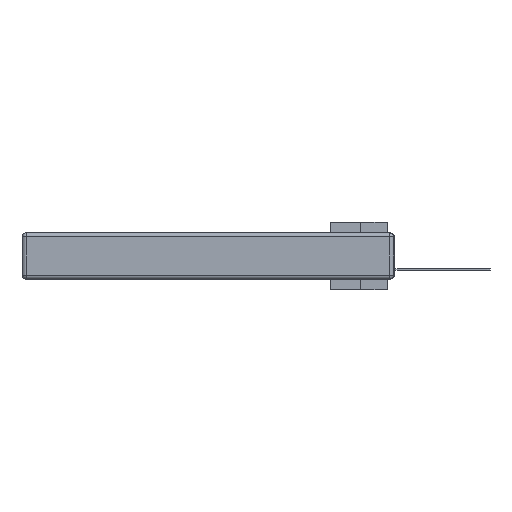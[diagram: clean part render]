
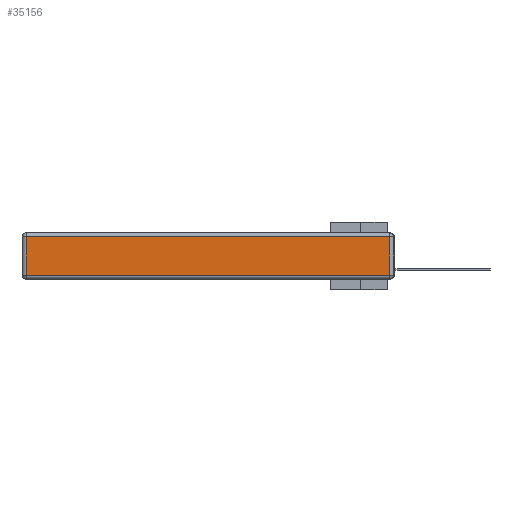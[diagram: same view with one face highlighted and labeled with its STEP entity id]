
A CAD part, left-side view. The second image highlights one B-rep face of the part: STEP entity #35156.
In plain terms, the highlighted planar face has unit normal (-1, 0, 0).
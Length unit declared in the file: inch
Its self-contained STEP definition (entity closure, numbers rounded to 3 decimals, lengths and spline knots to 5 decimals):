
#4 = EDGE_LOOP ( 'NONE', ( #25495, #147, #32077, #815 ) ) ;
#147 = ORIENTED_EDGE ( 'NONE', *, *, #21428, .T. ) ;
#815 = ORIENTED_EDGE ( 'NONE', *, *, #32978, .T. ) ;
#996 = LINE ( 'NONE', #24445, #1953 ) ;
#1953 = VECTOR ( 'NONE', #3888, 39.37008 ) ;
#2244 = AXIS2_PLACEMENT_3D ( 'NONE', #6804, #35891, #18681 ) ;
#3125 = CARTESIAN_POINT ( 'NONE',  ( 0., 2.72, -0.313 ) ) ;
#3888 = DIRECTION ( 'NONE',  ( 0., 1., 0. ) ) ;
#5013 = VECTOR ( 'NONE', #20433, 39.37008 ) ;
#5311 = CARTESIAN_POINT ( 'NONE',  ( 0., 0.03, -0.343 ) ) ;
#6804 = CARTESIAN_POINT ( 'NONE',  ( 0., 0., -0.343 ) ) ;
#7514 = LINE ( 'NONE', #17478, #15366 ) ;
#7903 = CARTESIAN_POINT ( 'NONE',  ( 0., 0.03, -0.313 ) ) ;
#8683 = VERTEX_POINT ( 'NONE', #11463 ) ;
#10481 = FACE_OUTER_BOUND ( 'NONE', #4, .T. ) ;
#11463 = CARTESIAN_POINT ( 'NONE',  ( 0., 0.03, -0.03 ) ) ;
#13597 = EDGE_CURVE ( 'NONE', #29920, #30816, #7514, .T. ) ;
#15366 = VECTOR ( 'NONE', #32072, 39.37008 ) ;
#15825 = VERTEX_POINT ( 'NONE', #30390 ) ;
#17478 = CARTESIAN_POINT ( 'NONE',  ( 0., 0., -0.313 ) ) ;
#18681 = DIRECTION ( 'NONE',  ( 0., 0., 1. ) ) ;
#20433 = DIRECTION ( 'NONE',  ( 0., 0., -1. ) ) ;
#20691 = LINE ( 'NONE', #34731, #5013 ) ;
#21174 = LINE ( 'NONE', #5311, #36451 ) ;
#21428 = EDGE_CURVE ( 'NONE', #30816, #8683, #21174, .T. ) ;
#22908 = DIRECTION ( 'NONE',  ( 0., 0., 1. ) ) ;
#24445 = CARTESIAN_POINT ( 'NONE',  ( 0., 2.75, -0.03 ) ) ;
#25300 = EDGE_CURVE ( 'NONE', #8683, #15825, #996, .T. ) ;
#25495 = ORIENTED_EDGE ( 'NONE', *, *, #13597, .T. ) ;
#29920 = VERTEX_POINT ( 'NONE', #3125 ) ;
#30390 = CARTESIAN_POINT ( 'NONE',  ( 0., 2.72, -0.03 ) ) ;
#30816 = VERTEX_POINT ( 'NONE', #7903 ) ;
#32072 = DIRECTION ( 'NONE',  ( 0., -1., 0. ) ) ;
#32077 = ORIENTED_EDGE ( 'NONE', *, *, #25300, .T. ) ;
#32978 = EDGE_CURVE ( 'NONE', #15825, #29920, #20691, .T. ) ;
#33000 = PLANE ( 'NONE',  #2244 ) ;
#34731 = CARTESIAN_POINT ( 'NONE',  ( 0., 2.72, -0.343 ) ) ;
#35156 = ADVANCED_FACE ( 'NONE', ( #10481 ), #33000, .T. ) ;
#35891 = DIRECTION ( 'NONE',  ( -1., 0., 0. ) ) ;
#36451 = VECTOR ( 'NONE', #22908, 39.37008 ) ;
